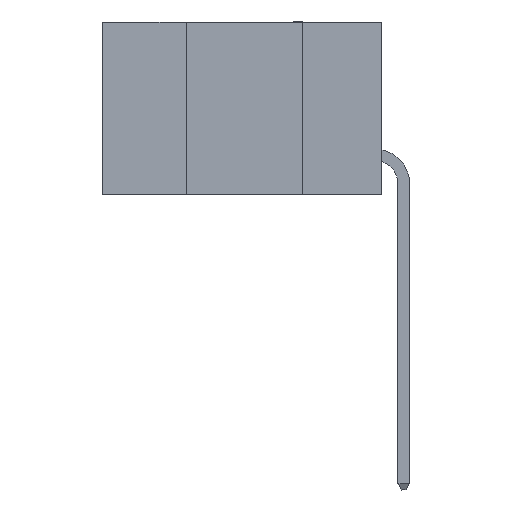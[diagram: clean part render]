
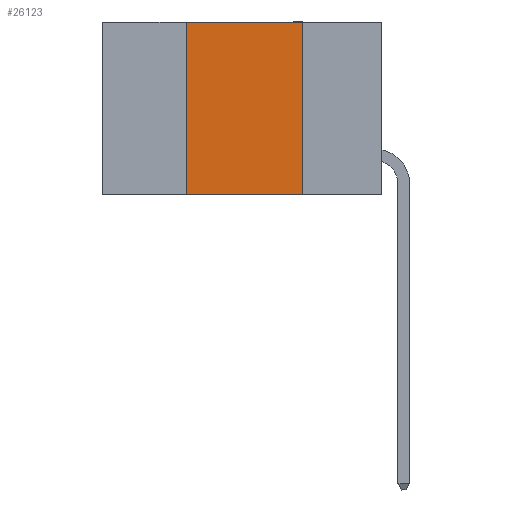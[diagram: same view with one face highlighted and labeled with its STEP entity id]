
A CAD part, left-side view. The second image highlights one B-rep face of the part: STEP entity #26123.
In plain terms, the highlighted planar face has unit normal (-1, 0, 0).
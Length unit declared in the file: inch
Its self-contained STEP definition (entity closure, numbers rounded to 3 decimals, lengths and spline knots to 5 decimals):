
#931 = CARTESIAN_POINT ( 'NONE',  ( 0., 0.17, -0.37 ) ) ;
#1622 = CARTESIAN_POINT ( 'NONE',  ( 0., 0.42, -0.37 ) ) ;
#4308 = VERTEX_POINT ( 'NONE', #1622 ) ;
#4682 = VECTOR ( 'NONE', #24593, 39.37008 ) ;
#5467 = VERTEX_POINT ( 'NONE', #931 ) ;
#7952 = EDGE_CURVE ( 'NONE', #4308, #5467, #10773, .T. ) ;
#8479 = CARTESIAN_POINT ( 'NONE',  ( 0., 0.42, 0. ) ) ;
#9159 = VECTOR ( 'NONE', #21959, 39.37008 ) ;
#9516 = EDGE_LOOP ( 'NONE', ( #11269, #26548, #9599, #12373 ) ) ;
#9599 = ORIENTED_EDGE ( 'NONE', *, *, #13869, .F. ) ;
#10773 = LINE ( 'NONE', #19332, #9159 ) ;
#11084 = DIRECTION ( 'NONE',  ( 0., 0., 1. ) ) ;
#11269 = ORIENTED_EDGE ( 'NONE', *, *, #12100, .F. ) ;
#11746 = LINE ( 'NONE', #16622, #4682 ) ;
#11971 = CARTESIAN_POINT ( 'NONE',  ( 0., 0.6, 0. ) ) ;
#12100 = EDGE_CURVE ( 'NONE', #30590, #5467, #11746, .T. ) ;
#12373 = ORIENTED_EDGE ( 'NONE', *, *, #7952, .T. ) ;
#12412 = FACE_OUTER_BOUND ( 'NONE', #9516, .T. ) ;
#12576 = DIRECTION ( 'NONE',  ( 0., 0., -1. ) ) ;
#13869 = EDGE_CURVE ( 'NONE', #4308, #16256, #17029, .T. ) ;
#14081 = EDGE_CURVE ( 'NONE', #16256, #30590, #15774, .T. ) ;
#15774 = LINE ( 'NONE', #11971, #21937 ) ;
#16256 = VERTEX_POINT ( 'NONE', #23636 ) ;
#16622 = CARTESIAN_POINT ( 'NONE',  ( 0., 0.17, 0. ) ) ;
#17029 = LINE ( 'NONE', #8479, #29494 ) ;
#19332 = CARTESIAN_POINT ( 'NONE',  ( 0., 0.6, -0.37 ) ) ;
#21937 = VECTOR ( 'NONE', #33143, 39.37008 ) ;
#21959 = DIRECTION ( 'NONE',  ( 0., -1., 0. ) ) ;
#23636 = CARTESIAN_POINT ( 'NONE',  ( 0., 0.42, 0. ) ) ;
#24593 = DIRECTION ( 'NONE',  ( 0., 0., -1. ) ) ;
#25738 = AXIS2_PLACEMENT_3D ( 'NONE', #31017, #28449, #12576 ) ;
#25767 = PLANE ( 'NONE',  #25738 ) ;
#26123 = ADVANCED_FACE ( 'NONE', ( #12412 ), #25767, .F. ) ;
#26548 = ORIENTED_EDGE ( 'NONE', *, *, #14081, .F. ) ;
#28449 = DIRECTION ( 'NONE',  ( 1., 0., 0. ) ) ;
#29494 = VECTOR ( 'NONE', #11084, 39.37008 ) ;
#30590 = VERTEX_POINT ( 'NONE', #33766 ) ;
#31017 = CARTESIAN_POINT ( 'NONE',  ( 0., 0.6, 0. ) ) ;
#33143 = DIRECTION ( 'NONE',  ( 0., -1., 0. ) ) ;
#33766 = CARTESIAN_POINT ( 'NONE',  ( 0., 0.17, 0. ) ) ;
